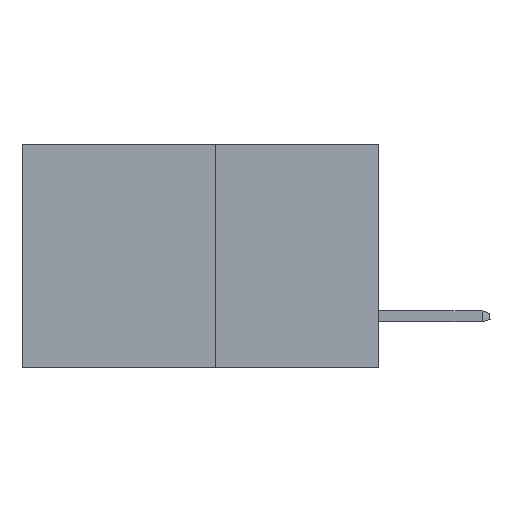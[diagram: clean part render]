
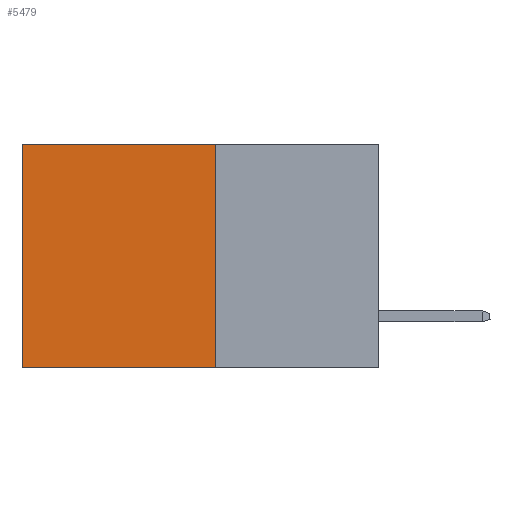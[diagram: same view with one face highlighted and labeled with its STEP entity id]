
A CAD part, left-side view. The second image highlights one B-rep face of the part: STEP entity #5479.
In plain terms, the highlighted planar face has unit normal (-1, 0, 0).
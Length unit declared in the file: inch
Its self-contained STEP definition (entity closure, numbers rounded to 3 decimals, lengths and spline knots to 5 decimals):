
#333 = CARTESIAN_POINT ( 'NONE',  ( 0.277, 0.27, -0.37 ) ) ;
#581 = CARTESIAN_POINT ( 'NONE',  ( 0.277, 0.27, 0. ) ) ;
#616 = DIRECTION ( 'NONE',  ( 0., 0., -1. ) ) ;
#622 = DIRECTION ( 'NONE',  ( 1., 0., 0. ) ) ;
#1011 = PLANE ( 'NONE',  #9318 ) ;
#1067 = CARTESIAN_POINT ( 'NONE',  ( 0.277, 0.27, -0.37 ) ) ;
#1709 = DIRECTION ( 'NONE',  ( 0., 1., 0. ) ) ;
#2280 = DIRECTION ( 'NONE',  ( 0., 0., -1. ) ) ;
#2804 = VECTOR ( 'NONE', #9956, 39.37008 ) ;
#2811 = VECTOR ( 'NONE', #1709, 39.37008 ) ;
#3237 = EDGE_LOOP ( 'NONE', ( #7919, #13248, #5454, #5798 ) ) ;
#3872 = VERTEX_POINT ( 'NONE', #3906 ) ;
#3906 = CARTESIAN_POINT ( 'NONE',  ( 0.277, 0.27, 0. ) ) ;
#4480 = CARTESIAN_POINT ( 'NONE',  ( 0.277, 0.27, -0.37 ) ) ;
#4794 = CARTESIAN_POINT ( 'NONE',  ( 0.277, 0.27, -0.37 ) ) ;
#5454 = ORIENTED_EDGE ( 'NONE', *, *, #7135, .F. ) ;
#5479 = ADVANCED_FACE ( 'NONE', ( #10583 ), #1011, .F. ) ;
#5673 = LINE ( 'NONE', #333, #2804 ) ;
#5798 = ORIENTED_EDGE ( 'NONE', *, *, #10789, .T. ) ;
#6509 = VECTOR ( 'NONE', #12981, 39.37008 ) ;
#7023 = CARTESIAN_POINT ( 'NONE',  ( 0.277, 0.59, 0. ) ) ;
#7093 = VECTOR ( 'NONE', #2280, 39.37008 ) ;
#7135 = EDGE_CURVE ( 'NONE', #3872, #9753, #11940, .T. ) ;
#7919 = ORIENTED_EDGE ( 'NONE', *, *, #12597, .T. ) ;
#8314 = EDGE_CURVE ( 'NONE', #9753, #13375, #5673, .T. ) ;
#8749 = VERTEX_POINT ( 'NONE', #7023 ) ;
#9318 = AXIS2_PLACEMENT_3D ( 'NONE', #1067, #622, #616 ) ;
#9673 = CARTESIAN_POINT ( 'NONE',  ( 0.277, 0.59, -0.37 ) ) ;
#9753 = VERTEX_POINT ( 'NONE', #4480 ) ;
#9824 = LINE ( 'NONE', #9673, #7093 ) ;
#9956 = DIRECTION ( 'NONE',  ( 0., 1., 0. ) ) ;
#10583 = FACE_OUTER_BOUND ( 'NONE', #3237, .T. ) ;
#10722 = CARTESIAN_POINT ( 'NONE',  ( 0.277, 0.59, -0.37 ) ) ;
#10789 = EDGE_CURVE ( 'NONE', #3872, #8749, #13147, .T. ) ;
#11940 = LINE ( 'NONE', #4794, #6509 ) ;
#12597 = EDGE_CURVE ( 'NONE', #8749, #13375, #9824, .T. ) ;
#12981 = DIRECTION ( 'NONE',  ( 0., 0., -1. ) ) ;
#13147 = LINE ( 'NONE', #581, #2811 ) ;
#13248 = ORIENTED_EDGE ( 'NONE', *, *, #8314, .F. ) ;
#13375 = VERTEX_POINT ( 'NONE', #10722 ) ;
